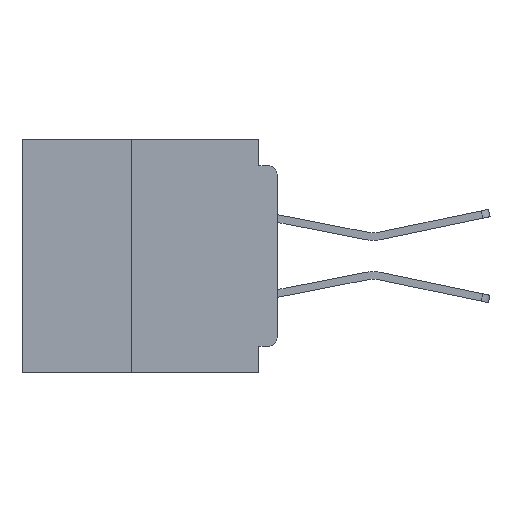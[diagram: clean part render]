
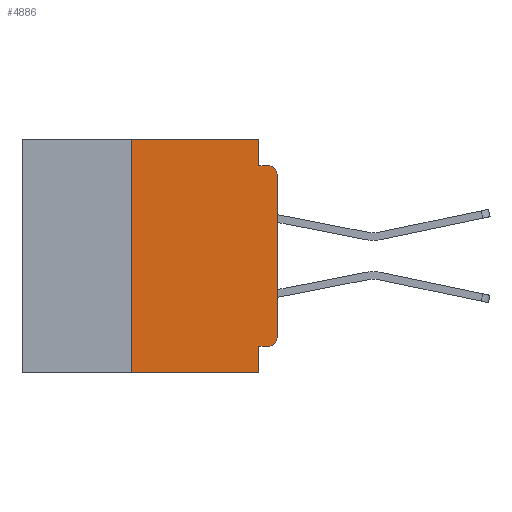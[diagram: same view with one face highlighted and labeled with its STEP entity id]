
A CAD part, left-side view. The second image highlights one B-rep face of the part: STEP entity #4886.
In plain terms, the highlighted planar face has unit normal (-1, 0, 0).
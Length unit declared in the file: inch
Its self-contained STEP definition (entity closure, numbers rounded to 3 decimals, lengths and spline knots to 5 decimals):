
#463 = ORIENTED_EDGE ( 'NONE', *, *, #42074, .F. ) ;
#817 = CARTESIAN_POINT ( 'NONE',  ( 0., 0.437, 0. ) ) ;
#921 = PLANE ( 'NONE',  #39214 ) ;
#2896 = VECTOR ( 'NONE', #15534, 39.37008 ) ;
#3054 = ORIENTED_EDGE ( 'NONE', *, *, #12813, .T. ) ;
#3397 = VECTOR ( 'NONE', #29154, 39.37008 ) ;
#3512 = DIRECTION ( 'NONE',  ( -1., 0., 0. ) ) ;
#3899 = CARTESIAN_POINT ( 'NONE',  ( 0., 0.031, -0.4 ) ) ;
#3913 = LINE ( 'NONE', #9913, #41875 ) ;
#4024 = LINE ( 'NONE', #32739, #2896 ) ;
#4886 = ADVANCED_FACE ( 'NONE', ( #35481 ), #921, .F. ) ;
#5900 = EDGE_LOOP ( 'NONE', ( #8951, #10439, #37844, #41210, #43833, #26239, #3054, #463, #8377, #21636 ) ) ;
#6016 = VECTOR ( 'NONE', #35354, 39.37008 ) ;
#8287 = CARTESIAN_POINT ( 'NONE',  ( 0., 0.031, 0. ) ) ;
#8377 = ORIENTED_EDGE ( 'NONE', *, *, #20025, .F. ) ;
#8664 = CIRCLE ( 'NONE', #9017, 0.015 ) ;
#8682 = CARTESIAN_POINT ( 'NONE',  ( 0., 0.437, -0.4 ) ) ;
#8951 = ORIENTED_EDGE ( 'NONE', *, *, #10666, .T. ) ;
#9017 = AXIS2_PLACEMENT_3D ( 'NONE', #32817, #12086, #36296 ) ;
#9913 = CARTESIAN_POINT ( 'NONE',  ( 0., 0., -0.045 ) ) ;
#10251 = LINE ( 'NONE', #3899, #26483 ) ;
#10439 = ORIENTED_EDGE ( 'NONE', *, *, #39863, .T. ) ;
#10666 = EDGE_CURVE ( 'NONE', #18424, #30417, #24433, .T. ) ;
#10911 = VERTEX_POINT ( 'NONE', #19441 ) ;
#12086 = DIRECTION ( 'NONE',  ( -1., 0., 0. ) ) ;
#12813 = EDGE_CURVE ( 'NONE', #39093, #35184, #36270, .T. ) ;
#14066 = VERTEX_POINT ( 'NONE', #15533 ) ;
#14857 = CARTESIAN_POINT ( 'NONE',  ( 0., 0.031, 0. ) ) ;
#15097 = VERTEX_POINT ( 'NONE', #17391 ) ;
#15102 = VECTOR ( 'NONE', #35545, 39.37008 ) ;
#15444 = CARTESIAN_POINT ( 'NONE',  ( 0., 0., -0.355 ) ) ;
#15533 = CARTESIAN_POINT ( 'NONE',  ( 0., 0.015, -0.355 ) ) ;
#15534 = DIRECTION ( 'NONE',  ( 0., 0., 1. ) ) ;
#15589 = EDGE_CURVE ( 'NONE', #10911, #30275, #3913, .T. ) ;
#16793 = VECTOR ( 'NONE', #32910, 39.37008 ) ;
#17391 = CARTESIAN_POINT ( 'NONE',  ( 0., 0.25, 0. ) ) ;
#18339 = CARTESIAN_POINT ( 'NONE',  ( 0., 0.031, -0.355 ) ) ;
#18424 = VERTEX_POINT ( 'NONE', #36415 ) ;
#18534 = DIRECTION ( 'NONE',  ( 1., 0., 0. ) ) ;
#19441 = CARTESIAN_POINT ( 'NONE',  ( 0., 0.031, -0.045 ) ) ;
#20025 = EDGE_CURVE ( 'NONE', #14066, #24292, #31168, .T. ) ;
#20326 = CARTESIAN_POINT ( 'NONE',  ( 0., 0.25, -0.4 ) ) ;
#21636 = ORIENTED_EDGE ( 'NONE', *, *, #22415, .T. ) ;
#22092 = CARTESIAN_POINT ( 'NONE',  ( 0., 0.015, -0.045 ) ) ;
#22415 = EDGE_CURVE ( 'NONE', #14066, #18424, #36445, .T. ) ;
#22798 = LINE ( 'NONE', #817, #23879 ) ;
#23879 = VECTOR ( 'NONE', #25222, 39.37008 ) ;
#24292 = VERTEX_POINT ( 'NONE', #18339 ) ;
#24355 = CARTESIAN_POINT ( 'NONE',  ( 0., 0.015, -0.34 ) ) ;
#24433 = LINE ( 'NONE', #31875, #6016 ) ;
#25009 = EDGE_CURVE ( 'NONE', #15097, #32280, #22798, .T. ) ;
#25222 = DIRECTION ( 'NONE',  ( 0., -1., 0. ) ) ;
#25307 = LINE ( 'NONE', #14857, #15102 ) ;
#26239 = ORIENTED_EDGE ( 'NONE', *, *, #27716, .F. ) ;
#26483 = VECTOR ( 'NONE', #31723, 39.37008 ) ;
#26997 = EDGE_CURVE ( 'NONE', #32280, #10911, #25307, .T. ) ;
#27716 = EDGE_CURVE ( 'NONE', #39093, #15097, #4024, .T. ) ;
#27844 = DIRECTION ( 'NONE',  ( 0., 0., -1. ) ) ;
#29002 = CARTESIAN_POINT ( 'NONE',  ( 0., 0.031, -0.4 ) ) ;
#29154 = DIRECTION ( 'NONE',  ( 0., 1., 0. ) ) ;
#30275 = VERTEX_POINT ( 'NONE', #22092 ) ;
#30417 = VERTEX_POINT ( 'NONE', #43624 ) ;
#31168 = LINE ( 'NONE', #15444, #3397 ) ;
#31723 = DIRECTION ( 'NONE',  ( 0., 0., -1. ) ) ;
#31875 = CARTESIAN_POINT ( 'NONE',  ( 0., 0., 0. ) ) ;
#32280 = VERTEX_POINT ( 'NONE', #8287 ) ;
#32739 = CARTESIAN_POINT ( 'NONE',  ( 0., 0.25, -0.4 ) ) ;
#32817 = CARTESIAN_POINT ( 'NONE',  ( 0., 0.015, -0.06 ) ) ;
#32910 = DIRECTION ( 'NONE',  ( 0., -1., 0. ) ) ;
#34127 = DIRECTION ( 'NONE',  ( 0., -1., 0. ) ) ;
#35184 = VERTEX_POINT ( 'NONE', #29002 ) ;
#35354 = DIRECTION ( 'NONE',  ( 0., 0., 1. ) ) ;
#35481 = FACE_OUTER_BOUND ( 'NONE', #5900, .T. ) ;
#35545 = DIRECTION ( 'NONE',  ( 0., 0., -1. ) ) ;
#36270 = LINE ( 'NONE', #8682, #16793 ) ;
#36296 = DIRECTION ( 'NONE',  ( 0., 0., -1. ) ) ;
#36415 = CARTESIAN_POINT ( 'NONE',  ( 0., 0., -0.34 ) ) ;
#36445 = CIRCLE ( 'NONE', #44515, 0.015 ) ;
#37844 = ORIENTED_EDGE ( 'NONE', *, *, #15589, .F. ) ;
#39093 = VERTEX_POINT ( 'NONE', #20326 ) ;
#39214 = AXIS2_PLACEMENT_3D ( 'NONE', #39226, #18534, #42665 ) ;
#39226 = CARTESIAN_POINT ( 'NONE',  ( 0., 0.437, 0. ) ) ;
#39863 = EDGE_CURVE ( 'NONE', #30417, #30275, #8664, .T. ) ;
#41210 = ORIENTED_EDGE ( 'NONE', *, *, #26997, .F. ) ;
#41875 = VECTOR ( 'NONE', #34127, 39.37008 ) ;
#42074 = EDGE_CURVE ( 'NONE', #24292, #35184, #10251, .T. ) ;
#42665 = DIRECTION ( 'NONE',  ( 0., 0., -1. ) ) ;
#43624 = CARTESIAN_POINT ( 'NONE',  ( 0., 0., -0.06 ) ) ;
#43833 = ORIENTED_EDGE ( 'NONE', *, *, #25009, .F. ) ;
#44515 = AXIS2_PLACEMENT_3D ( 'NONE', #24355, #3512, #27844 ) ;
